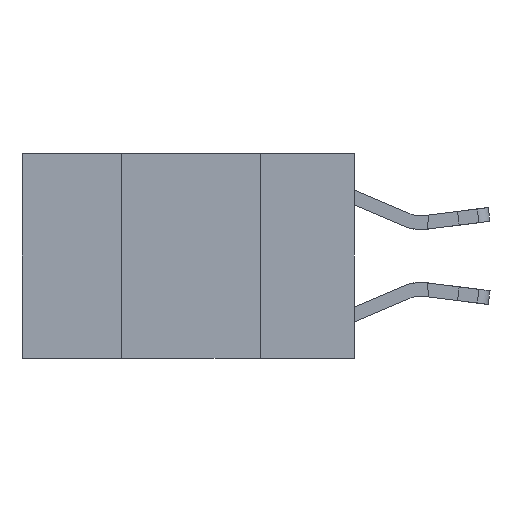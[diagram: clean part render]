
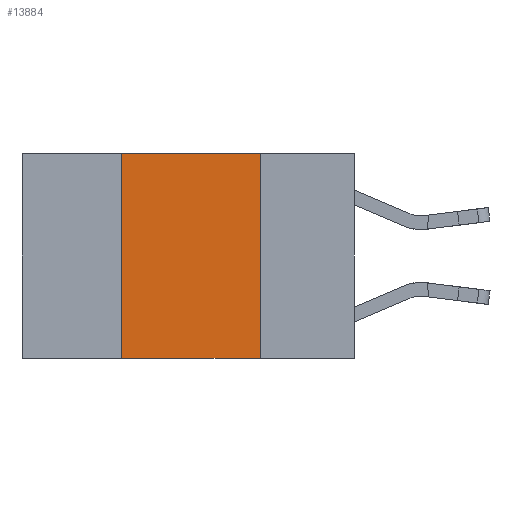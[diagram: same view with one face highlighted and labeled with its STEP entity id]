
A CAD part, left-side view. The second image highlights one B-rep face of the part: STEP entity #13884.
In plain terms, the highlighted planar face has unit normal (-1, 0, 0).
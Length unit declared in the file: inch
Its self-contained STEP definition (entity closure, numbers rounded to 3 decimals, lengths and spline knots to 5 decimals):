
#247 = EDGE_CURVE ( 'NONE', #7177, #19345, #2418, .T. ) ;
#690 = CARTESIAN_POINT ( 'NONE',  ( 0., 0.42, 0. ) ) ;
#1975 = VERTEX_POINT ( 'NONE', #6810 ) ;
#2418 = LINE ( 'NONE', #5684, #4146 ) ;
#2497 = VERTEX_POINT ( 'NONE', #18920 ) ;
#4146 = VECTOR ( 'NONE', #17078, 39.37008 ) ;
#4489 = ORIENTED_EDGE ( 'NONE', *, *, #20564, .F. ) ;
#4739 = PLANE ( 'NONE',  #7995 ) ;
#5684 = CARTESIAN_POINT ( 'NONE',  ( 0., 0.42, 0. ) ) ;
#6401 = DIRECTION ( 'NONE',  ( 0., -1., 0. ) ) ;
#6810 = CARTESIAN_POINT ( 'NONE',  ( 0., 0.17, 0. ) ) ;
#6837 = EDGE_CURVE ( 'NONE', #7177, #2497, #20764, .T. ) ;
#7177 = VERTEX_POINT ( 'NONE', #18838 ) ;
#7694 = ORIENTED_EDGE ( 'NONE', *, *, #6837, .T. ) ;
#7888 = DIRECTION ( 'NONE',  ( 1., 0., 0. ) ) ;
#7899 = CARTESIAN_POINT ( 'NONE',  ( 0., 0.6, -0.37 ) ) ;
#7995 = AXIS2_PLACEMENT_3D ( 'NONE', #16131, #7888, #19282 ) ;
#9702 = VECTOR ( 'NONE', #10292, 39.37008 ) ;
#10292 = DIRECTION ( 'NONE',  ( 0., 0., -1. ) ) ;
#11146 = LINE ( 'NONE', #18954, #19305 ) ;
#11201 = VECTOR ( 'NONE', #19703, 39.37008 ) ;
#11314 = ORIENTED_EDGE ( 'NONE', *, *, #15635, .F. ) ;
#11879 = LINE ( 'NONE', #18315, #9702 ) ;
#13884 = ADVANCED_FACE ( 'NONE', ( #18450 ), #4739, .F. ) ;
#14342 = EDGE_LOOP ( 'NONE', ( #4489, #11314, #19985, #7694 ) ) ;
#15635 = EDGE_CURVE ( 'NONE', #19345, #1975, #11146, .T. ) ;
#16131 = CARTESIAN_POINT ( 'NONE',  ( 0., 0.6, 0. ) ) ;
#17078 = DIRECTION ( 'NONE',  ( 0., 0., 1. ) ) ;
#18315 = CARTESIAN_POINT ( 'NONE',  ( 0., 0.17, 0. ) ) ;
#18450 = FACE_OUTER_BOUND ( 'NONE', #14342, .T. ) ;
#18838 = CARTESIAN_POINT ( 'NONE',  ( 0., 0.42, -0.37 ) ) ;
#18920 = CARTESIAN_POINT ( 'NONE',  ( 0., 0.17, -0.37 ) ) ;
#18954 = CARTESIAN_POINT ( 'NONE',  ( 0., 0.6, 0. ) ) ;
#19282 = DIRECTION ( 'NONE',  ( 0., 0., -1. ) ) ;
#19305 = VECTOR ( 'NONE', #6401, 39.37008 ) ;
#19345 = VERTEX_POINT ( 'NONE', #690 ) ;
#19703 = DIRECTION ( 'NONE',  ( 0., -1., 0. ) ) ;
#19985 = ORIENTED_EDGE ( 'NONE', *, *, #247, .F. ) ;
#20564 = EDGE_CURVE ( 'NONE', #1975, #2497, #11879, .T. ) ;
#20764 = LINE ( 'NONE', #7899, #11201 ) ;
